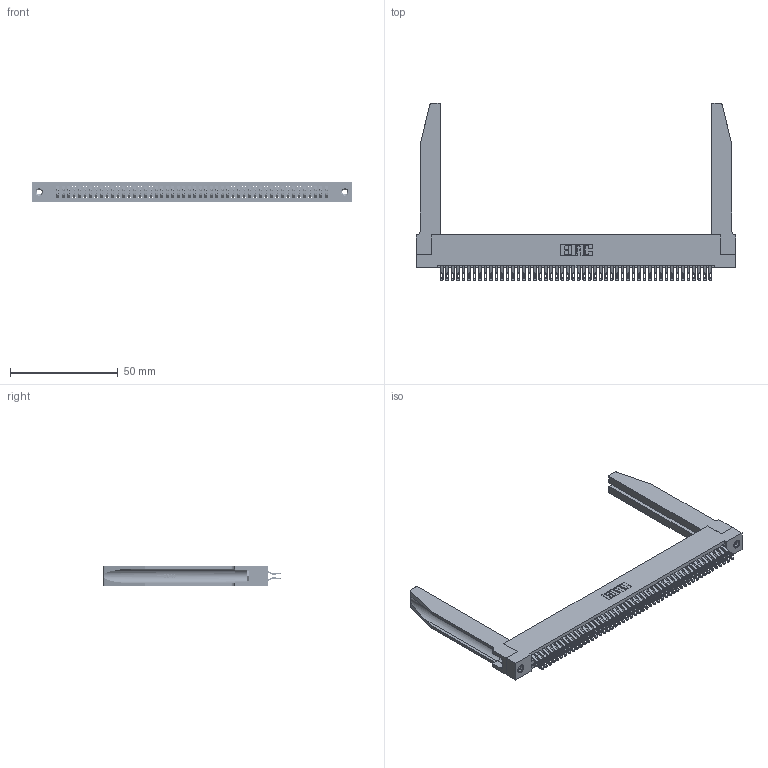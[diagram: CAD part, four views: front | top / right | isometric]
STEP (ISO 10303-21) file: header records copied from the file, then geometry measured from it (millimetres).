
FILE_DESCRIPTION (( 'STEP AP203' ), '1' );
FILE_NAME ('395-100-555-278.STEP', '2019-10-26T16:13:17', ( '' ), ( '' ), 'SwSTEP 2.0', 'SolidWorks 2016', '' );
FILE_SCHEMA (( 'CONFIG_CONTROL_DESIGN' ));
Length unit declared in the file: inch
Products named in the file (5): 345 Part_Flush Mounting Lugs - 0.156 Dia-TH; 345-292-001_555 Tail; 345-250-001_345-250-001-102; 345-220-078_345-220-078; 395-100-555-278
Assembly tree (105 placements, depth 2):
  395-100-555-278
    345 Part_Flush Mounting Lugs - 0.156 Dia-TH
    345-292-001_555 Tail  x100
    345-250-001_345-250-001-102  x2
    345-220-078_345-220-078  x2
Bounding box: 148.23 x 82.09 x 9.4 mm (x, y, z)
Volume: 22534.4 mm3; surface area: 29825.8 mm2
Topology: 105 solids, 105 shells, 5960 faces, 18649 edges, 12422 vertices
Faces by surface type: plane 3322, cylinder 2586, bspline 36, cone 12, torus 4
Entity records: 43220 total; most frequent: CARTESIAN_POINT 8189, ORIENTED_EDGE 6990, DIRECTION 6173, EDGE_CURVE 3495, VECTOR 3049, LINE 3049, VERTEX_POINT 2324, AXIS2_PLACEMENT_3D 1562
